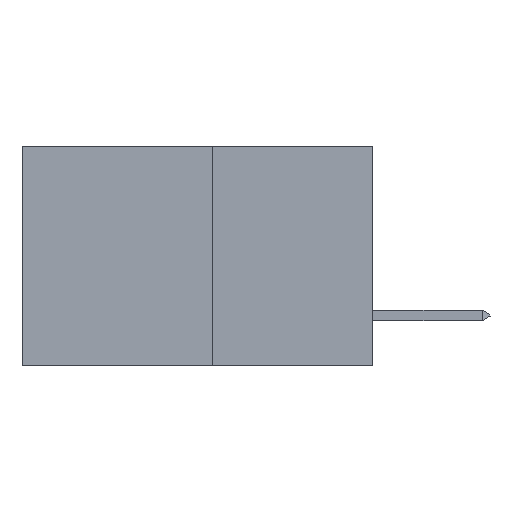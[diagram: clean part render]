
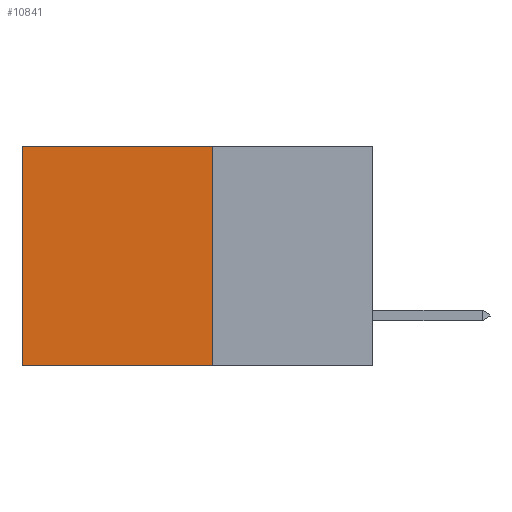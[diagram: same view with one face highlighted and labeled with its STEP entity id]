
A CAD part, left-side view. The second image highlights one B-rep face of the part: STEP entity #10841.
In plain terms, the highlighted planar face has unit normal (-1, 0, 0).
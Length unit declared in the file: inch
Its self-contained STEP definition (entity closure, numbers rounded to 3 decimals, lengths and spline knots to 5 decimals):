
#238 = VERTEX_POINT ( 'NONE', #1525 ) ;
#809 = DIRECTION ( 'NONE',  ( 0., 1., 0. ) ) ;
#1036 = EDGE_CURVE ( 'NONE', #8636, #1685, #10181, .T. ) ;
#1482 = CARTESIAN_POINT ( 'NONE',  ( 0.277, 0.59, -0.37 ) ) ;
#1525 = CARTESIAN_POINT ( 'NONE',  ( 0.277, 0.27, 0. ) ) ;
#1633 = AXIS2_PLACEMENT_3D ( 'NONE', #13638, #6638, #14705 ) ;
#1685 = VERTEX_POINT ( 'NONE', #1482 ) ;
#2115 = EDGE_CURVE ( 'NONE', #8424, #1685, #7318, .T. ) ;
#2506 = ORIENTED_EDGE ( 'NONE', *, *, #13733, .T. ) ;
#2671 = LINE ( 'NONE', #4581, #6035 ) ;
#3283 = DIRECTION ( 'NONE',  ( 0., 1., 0. ) ) ;
#3761 = VECTOR ( 'NONE', #809, 39.37008 ) ;
#3901 = EDGE_CURVE ( 'NONE', #238, #8636, #7590, .T. ) ;
#4021 = VECTOR ( 'NONE', #7987, 39.37008 ) ;
#4581 = CARTESIAN_POINT ( 'NONE',  ( 0.277, 0.27, 0. ) ) ;
#5389 = PLANE ( 'NONE',  #1633 ) ;
#5502 = CARTESIAN_POINT ( 'NONE',  ( 0.277, 0.59, 0. ) ) ;
#6035 = VECTOR ( 'NONE', #3283, 39.37008 ) ;
#6265 = ORIENTED_EDGE ( 'NONE', *, *, #2115, .T. ) ;
#6638 = DIRECTION ( 'NONE',  ( 1., 0., 0. ) ) ;
#7318 = LINE ( 'NONE', #14418, #4021 ) ;
#7590 = LINE ( 'NONE', #11494, #13419 ) ;
#7987 = DIRECTION ( 'NONE',  ( 0., 0., -1. ) ) ;
#8076 = FACE_OUTER_BOUND ( 'NONE', #15328, .T. ) ;
#8214 = CARTESIAN_POINT ( 'NONE',  ( 0.277, 0.27, -0.37 ) ) ;
#8424 = VERTEX_POINT ( 'NONE', #5502 ) ;
#8636 = VERTEX_POINT ( 'NONE', #8214 ) ;
#10181 = LINE ( 'NONE', #14486, #3761 ) ;
#10841 = ADVANCED_FACE ( 'NONE', ( #8076 ), #5389, .F. ) ;
#11318 = DIRECTION ( 'NONE',  ( 0., 0., -1. ) ) ;
#11494 = CARTESIAN_POINT ( 'NONE',  ( 0.277, 0.27, -0.37 ) ) ;
#13419 = VECTOR ( 'NONE', #11318, 39.37008 ) ;
#13638 = CARTESIAN_POINT ( 'NONE',  ( 0.277, 0.27, -0.37 ) ) ;
#13733 = EDGE_CURVE ( 'NONE', #238, #8424, #2671, .T. ) ;
#14418 = CARTESIAN_POINT ( 'NONE',  ( 0.277, 0.59, -0.37 ) ) ;
#14443 = ORIENTED_EDGE ( 'NONE', *, *, #3901, .F. ) ;
#14486 = CARTESIAN_POINT ( 'NONE',  ( 0.277, 0.27, -0.37 ) ) ;
#14601 = ORIENTED_EDGE ( 'NONE', *, *, #1036, .F. ) ;
#14705 = DIRECTION ( 'NONE',  ( 0., 0., -1. ) ) ;
#15328 = EDGE_LOOP ( 'NONE', ( #6265, #14601, #14443, #2506 ) ) ;
